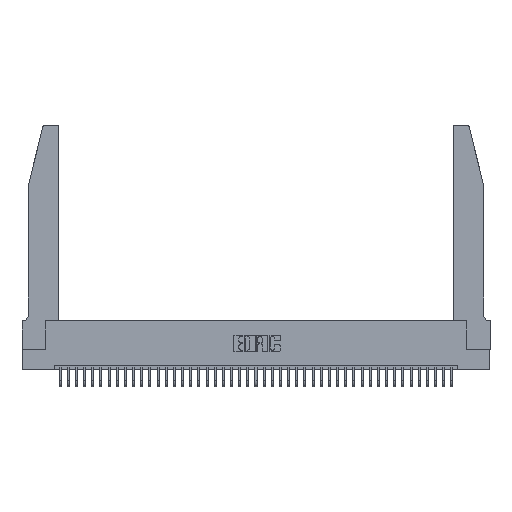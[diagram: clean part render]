
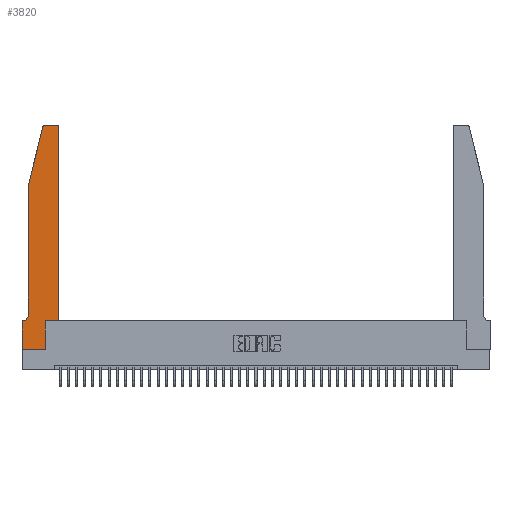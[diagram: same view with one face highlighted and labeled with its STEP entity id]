
A CAD part, top view. The second image highlights one B-rep face of the part: STEP entity #3820.
In plain terms, the highlighted planar face has unit normal (0, 0, 1).
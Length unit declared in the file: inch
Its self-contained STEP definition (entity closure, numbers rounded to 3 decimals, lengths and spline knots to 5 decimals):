
#206 = CARTESIAN_POINT ( 'NONE',  ( 0., 0., 0.37 ) ) ;
#357 = LINE ( 'NONE', #518, #34473 ) ;
#518 = CARTESIAN_POINT ( 'NONE',  ( 0.4505, 0.35, 0.37 ) ) ;
#632 = CARTESIAN_POINT ( 'NONE',  ( 0.0755, 2., 0.37 ) ) ;
#702 = LINE ( 'NONE', #7435, #9982 ) ;
#770 = FACE_OUTER_BOUND ( 'NONE', #30587, .T. ) ;
#1149 = DIRECTION ( 'NONE',  ( 1., 0., 0. ) ) ;
#1643 = ORIENTED_EDGE ( 'NONE', *, *, #33369, .T. ) ;
#1669 = CARTESIAN_POINT ( 'NONE',  ( 0.4505, 0.35, 0.37 ) ) ;
#3064 = CIRCLE ( 'NONE', #27860, 0.07 ) ;
#3694 = VERTEX_POINT ( 'NONE', #17650 ) ;
#3820 = ADVANCED_FACE ( 'NONE', ( #770 ), #42004, .T. ) ;
#3934 = VERTEX_POINT ( 'NONE', #42565 ) ;
#4425 = LINE ( 'NONE', #16607, #28419 ) ;
#4478 = VERTEX_POINT ( 'NONE', #8946 ) ;
#4729 = EDGE_CURVE ( 'NONE', #5886, #34409, #25870, .T. ) ;
#4773 = CARTESIAN_POINT ( 'NONE',  ( 0.4205, 2.75, 0.37 ) ) ;
#4839 = DIRECTION ( 'NONE',  ( 1., 0., 0. ) ) ;
#5886 = VERTEX_POINT ( 'NONE', #9911 ) ;
#6407 = VERTEX_POINT ( 'NONE', #19905 ) ;
#6678 = DIRECTION ( 'NONE',  ( 1., 0., 0. ) ) ;
#7369 = ORIENTED_EDGE ( 'NONE', *, *, #32410, .T. ) ;
#7435 = CARTESIAN_POINT ( 'NONE',  ( 0.0755, 0.35, 0.37 ) ) ;
#7540 = VECTOR ( 'NONE', #42304, 39.37008 ) ;
#7745 = ORIENTED_EDGE ( 'NONE', *, *, #42923, .T. ) ;
#7818 = CARTESIAN_POINT ( 'NONE',  ( 0.2605, 2.75, 0.37 ) ) ;
#8264 = CARTESIAN_POINT ( 'NONE',  ( 0.0055, 0.42, 0.37 ) ) ;
#8690 = CARTESIAN_POINT ( 'NONE',  ( 0.2865, 0.35, 0.37 ) ) ;
#8885 = VECTOR ( 'NONE', #23952, 39.37008 ) ;
#8946 = CARTESIAN_POINT ( 'NONE',  ( 0.25487, 2.72718, 0.37 ) ) ;
#9082 = LINE ( 'NONE', #8690, #43869 ) ;
#9899 = VECTOR ( 'NONE', #6678, 39.37008 ) ;
#9911 = CARTESIAN_POINT ( 'NONE',  ( 0., 0.35, 0.37 ) ) ;
#9982 = VECTOR ( 'NONE', #14300, 39.37008 ) ;
#10815 = VECTOR ( 'NONE', #11257, 39.37008 ) ;
#10844 = VERTEX_POINT ( 'NONE', #31488 ) ;
#11257 = DIRECTION ( 'NONE',  ( -1., 0., 0. ) ) ;
#11681 = DIRECTION ( 'NONE',  ( -1., 0., 0. ) ) ;
#13365 = CARTESIAN_POINT ( 'NONE',  ( 0.2865, 0., 0.37 ) ) ;
#13461 = VERTEX_POINT ( 'NONE', #42806 ) ;
#14112 = ORIENTED_EDGE ( 'NONE', *, *, #21873, .T. ) ;
#14257 = DIRECTION ( 'NONE',  ( 0., 1., 0. ) ) ;
#14300 = DIRECTION ( 'NONE',  ( -1., 0., 0. ) ) ;
#15788 = ORIENTED_EDGE ( 'NONE', *, *, #17006, .T. ) ;
#15811 = CIRCLE ( 'NONE', #22156, 0.03 ) ;
#16138 = CARTESIAN_POINT ( 'NONE',  ( 0.284, 2.72, 0.37 ) ) ;
#16607 = CARTESIAN_POINT ( 'NONE',  ( 0.0755, 2., 0.37 ) ) ;
#16727 = ORIENTED_EDGE ( 'NONE', *, *, #4729, .T. ) ;
#16901 = CARTESIAN_POINT ( 'NONE',  ( 0.0755, 2., 0.37 ) ) ;
#17006 = EDGE_CURVE ( 'NONE', #34409, #20378, #18988, .T. ) ;
#17650 = CARTESIAN_POINT ( 'NONE',  ( 0.4505, 0.35, 0.37 ) ) ;
#17722 = LINE ( 'NONE', #1669, #7540 ) ;
#18988 = LINE ( 'NONE', #40401, #9899 ) ;
#19626 = DIRECTION ( 'NONE',  ( 1., 0., 0. ) ) ;
#19905 = CARTESIAN_POINT ( 'NONE',  ( 0.4505, 2.72, 0.37 ) ) ;
#20073 = DIRECTION ( 'NONE',  ( -0.239, -0.971, 0. ) ) ;
#20378 = VERTEX_POINT ( 'NONE', #13365 ) ;
#21756 = EDGE_CURVE ( 'NONE', #3934, #5886, #702, .T. ) ;
#21785 = DIRECTION ( 'NONE',  ( 0., 0., 1. ) ) ;
#21873 = EDGE_CURVE ( 'NONE', #6407, #42400, #15811, .T. ) ;
#21963 = CARTESIAN_POINT ( 'NONE',  ( 0., 0.35, 0.37 ) ) ;
#22156 = AXIS2_PLACEMENT_3D ( 'NONE', #41824, #21785, #1149 ) ;
#22651 = ORIENTED_EDGE ( 'NONE', *, *, #31062, .T. ) ;
#23952 = DIRECTION ( 'NONE',  ( 0., -1., 0. ) ) ;
#25115 = VECTOR ( 'NONE', #41314, 39.37008 ) ;
#25238 = CARTESIAN_POINT ( 'NONE',  ( 0.0755, 0.42, 0.37 ) ) ;
#25298 = DIRECTION ( 'NONE',  ( 0., 0., 1. ) ) ;
#25870 = LINE ( 'NONE', #27736, #8885 ) ;
#27736 = CARTESIAN_POINT ( 'NONE',  ( 0., 0., 0.37 ) ) ;
#27860 = AXIS2_PLACEMENT_3D ( 'NONE', #8264, #31902, #11681 ) ;
#28419 = VECTOR ( 'NONE', #20073, 39.37008 ) ;
#28805 = LINE ( 'NONE', #7818, #10815 ) ;
#30587 = EDGE_LOOP ( 'NONE', ( #22651, #33633, #32803, #7745, #40791, #41506, #16727, #15788, #1643, #35083, #7369, #14112 ) ) ;
#30605 = LINE ( 'NONE', #632, #25115 ) ;
#31062 = EDGE_CURVE ( 'NONE', #42400, #10844, #28805, .T. ) ;
#31488 = CARTESIAN_POINT ( 'NONE',  ( 0.284, 2.75, 0.37 ) ) ;
#31902 = DIRECTION ( 'NONE',  ( 0., 0., -1. ) ) ;
#32169 = DIRECTION ( 'NONE',  ( 0., 1., 0. ) ) ;
#32410 = EDGE_CURVE ( 'NONE', #3694, #6407, #357, .T. ) ;
#32803 = ORIENTED_EDGE ( 'NONE', *, *, #36257, .T. ) ;
#33369 = EDGE_CURVE ( 'NONE', #20378, #13461, #9082, .T. ) ;
#33633 = ORIENTED_EDGE ( 'NONE', *, *, #41497, .T. ) ;
#34409 = VERTEX_POINT ( 'NONE', #206 ) ;
#34473 = VECTOR ( 'NONE', #14257, 39.37008 ) ;
#34638 = CIRCLE ( 'NONE', #35770, 0.03 ) ;
#35083 = ORIENTED_EDGE ( 'NONE', *, *, #43137, .T. ) ;
#35770 = AXIS2_PLACEMENT_3D ( 'NONE', #16138, #39696, #19626 ) ;
#36257 = EDGE_CURVE ( 'NONE', #4478, #36361, #4425, .T. ) ;
#36361 = VERTEX_POINT ( 'NONE', #16901 ) ;
#37836 = EDGE_CURVE ( 'NONE', #39155, #3934, #3064, .T. ) ;
#39155 = VERTEX_POINT ( 'NONE', #25238 ) ;
#39696 = DIRECTION ( 'NONE',  ( 0., 0., 1. ) ) ;
#40401 = CARTESIAN_POINT ( 'NONE',  ( 0., 0., 0.37 ) ) ;
#40791 = ORIENTED_EDGE ( 'NONE', *, *, #37836, .T. ) ;
#41314 = DIRECTION ( 'NONE',  ( 0., -1., 0. ) ) ;
#41497 = EDGE_CURVE ( 'NONE', #10844, #4478, #34638, .T. ) ;
#41506 = ORIENTED_EDGE ( 'NONE', *, *, #21756, .T. ) ;
#41824 = CARTESIAN_POINT ( 'NONE',  ( 0.4205, 2.72, 0.37 ) ) ;
#42004 = PLANE ( 'NONE',  #42525 ) ;
#42304 = DIRECTION ( 'NONE',  ( 1., 0., 0. ) ) ;
#42400 = VERTEX_POINT ( 'NONE', #4773 ) ;
#42525 = AXIS2_PLACEMENT_3D ( 'NONE', #21963, #25298, #4839 ) ;
#42565 = CARTESIAN_POINT ( 'NONE',  ( 0.0055, 0.35, 0.37 ) ) ;
#42806 = CARTESIAN_POINT ( 'NONE',  ( 0.2865, 0.35, 0.37 ) ) ;
#42923 = EDGE_CURVE ( 'NONE', #36361, #39155, #30605, .T. ) ;
#43137 = EDGE_CURVE ( 'NONE', #13461, #3694, #17722, .T. ) ;
#43869 = VECTOR ( 'NONE', #32169, 39.37008 ) ;
